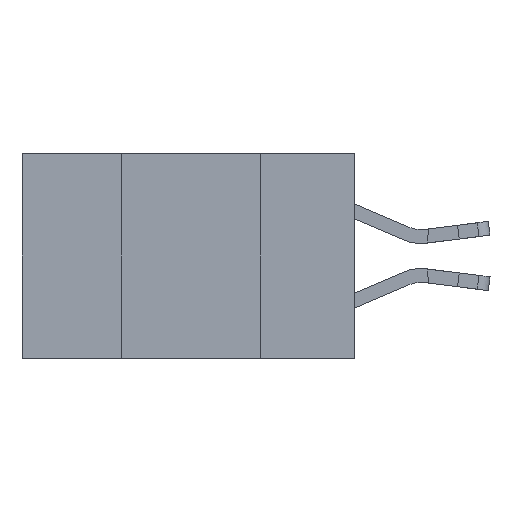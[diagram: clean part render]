
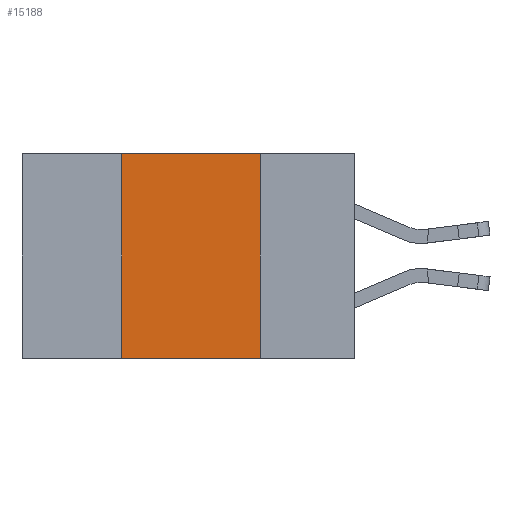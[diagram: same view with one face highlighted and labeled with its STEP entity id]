
A CAD part, left-side view. The second image highlights one B-rep face of the part: STEP entity #15188.
In plain terms, the highlighted planar face has unit normal (-1, 0, 0).
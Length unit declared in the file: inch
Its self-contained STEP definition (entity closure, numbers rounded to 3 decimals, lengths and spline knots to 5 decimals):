
#384 = LINE ( 'NONE', #12367, #2574 ) ;
#2374 = VERTEX_POINT ( 'NONE', #13275 ) ;
#2574 = VECTOR ( 'NONE', #4052, 39.37008 ) ;
#3895 = ORIENTED_EDGE ( 'NONE', *, *, #18190, .F. ) ;
#4052 = DIRECTION ( 'NONE',  ( 0., -1., 0. ) ) ;
#4221 = DIRECTION ( 'NONE',  ( 0., 0., 1. ) ) ;
#4417 = DIRECTION ( 'NONE',  ( 1., 0., 0. ) ) ;
#4521 = FACE_OUTER_BOUND ( 'NONE', #17836, .T. ) ;
#4600 = PLANE ( 'NONE',  #9809 ) ;
#5511 = ORIENTED_EDGE ( 'NONE', *, *, #10596, .F. ) ;
#5812 = DIRECTION ( 'NONE',  ( 0., 0., -1. ) ) ;
#6166 = CARTESIAN_POINT ( 'NONE',  ( 0., 0.17, 0. ) ) ;
#7154 = CARTESIAN_POINT ( 'NONE',  ( 0., 0.17, 0. ) ) ;
#7962 = CARTESIAN_POINT ( 'NONE',  ( 0., 0.6, -0.37 ) ) ;
#8417 = EDGE_CURVE ( 'NONE', #2374, #15905, #384, .T. ) ;
#8788 = CARTESIAN_POINT ( 'NONE',  ( 0., 0.6, 0. ) ) ;
#8917 = EDGE_CURVE ( 'NONE', #14815, #14371, #16594, .T. ) ;
#9809 = AXIS2_PLACEMENT_3D ( 'NONE', #8788, #4417, #5812 ) ;
#9824 = VECTOR ( 'NONE', #10781, 39.37008 ) ;
#10214 = ORIENTED_EDGE ( 'NONE', *, *, #8917, .T. ) ;
#10596 = EDGE_CURVE ( 'NONE', #15905, #14371, #10643, .T. ) ;
#10643 = LINE ( 'NONE', #7154, #16322 ) ;
#10781 = DIRECTION ( 'NONE',  ( 0., -1., 0. ) ) ;
#12367 = CARTESIAN_POINT ( 'NONE',  ( 0., 0.6, 0. ) ) ;
#12595 = CARTESIAN_POINT ( 'NONE',  ( 0., 0.42, 0. ) ) ;
#13275 = CARTESIAN_POINT ( 'NONE',  ( 0., 0.42, 0. ) ) ;
#14280 = DIRECTION ( 'NONE',  ( 0., 0., -1. ) ) ;
#14371 = VERTEX_POINT ( 'NONE', #16803 ) ;
#14560 = ORIENTED_EDGE ( 'NONE', *, *, #8417, .F. ) ;
#14815 = VERTEX_POINT ( 'NONE', #16261 ) ;
#15188 = ADVANCED_FACE ( 'NONE', ( #4521 ), #4600, .F. ) ;
#15560 = VECTOR ( 'NONE', #4221, 39.37008 ) ;
#15773 = LINE ( 'NONE', #12595, #15560 ) ;
#15905 = VERTEX_POINT ( 'NONE', #6166 ) ;
#16261 = CARTESIAN_POINT ( 'NONE',  ( 0., 0.42, -0.37 ) ) ;
#16322 = VECTOR ( 'NONE', #14280, 39.37008 ) ;
#16594 = LINE ( 'NONE', #7962, #9824 ) ;
#16803 = CARTESIAN_POINT ( 'NONE',  ( 0., 0.17, -0.37 ) ) ;
#17836 = EDGE_LOOP ( 'NONE', ( #5511, #14560, #3895, #10214 ) ) ;
#18190 = EDGE_CURVE ( 'NONE', #14815, #2374, #15773, .T. ) ;
